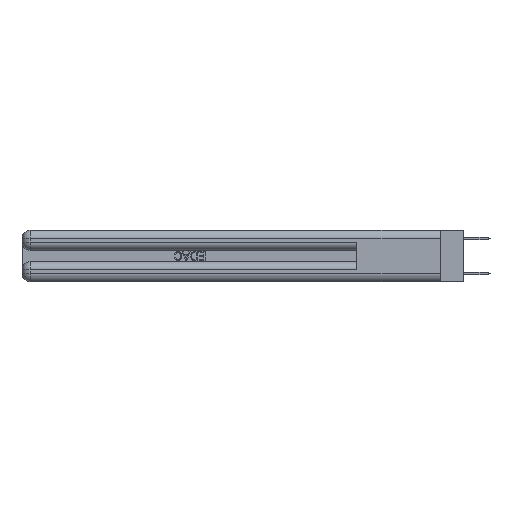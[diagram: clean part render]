
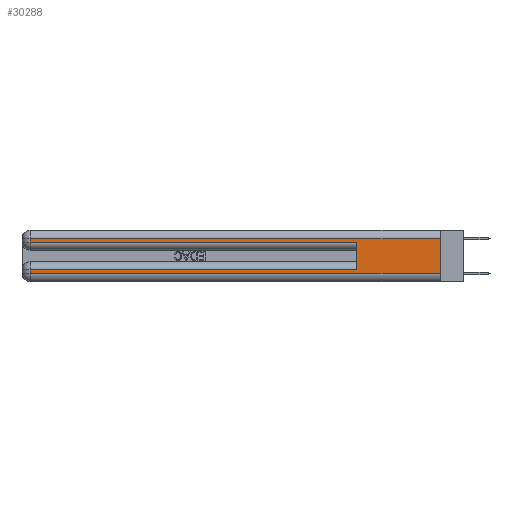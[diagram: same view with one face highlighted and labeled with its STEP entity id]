
A CAD part, left-side view. The second image highlights one B-rep face of the part: STEP entity #30288.
In plain terms, the highlighted planar face has unit normal (-1, 0, 0).
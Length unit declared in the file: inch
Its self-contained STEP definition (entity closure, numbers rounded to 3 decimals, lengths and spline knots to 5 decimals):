
#173 = ORIENTED_EDGE ( 'NONE', *, *, #21731, .T. ) ;
#549 = EDGE_CURVE ( 'NONE', #3078, #29532, #5573, .T. ) ;
#694 = VECTOR ( 'NONE', #29930, 39.37008 ) ;
#1896 = ORIENTED_EDGE ( 'NONE', *, *, #16696, .F. ) ;
#2566 = ORIENTED_EDGE ( 'NONE', *, *, #549, .F. ) ;
#2823 = DIRECTION ( 'NONE',  ( 0., 0., -1. ) ) ;
#3074 = CARTESIAN_POINT ( 'NONE',  ( 0., 0., 0.37 ) ) ;
#3078 = VERTEX_POINT ( 'NONE', #6567 ) ;
#3728 = DIRECTION ( 'NONE',  ( 0., 1., 0. ) ) ;
#4421 = VECTOR ( 'NONE', #19808, 39.37008 ) ;
#5366 = VECTOR ( 'NONE', #8567, 39.37008 ) ;
#5469 = PLANE ( 'NONE',  #11537 ) ;
#5573 = LINE ( 'NONE', #19978, #4421 ) ;
#5772 = LINE ( 'NONE', #10374, #694 ) ;
#5781 = DIRECTION ( 'NONE',  ( 0., 0., -1. ) ) ;
#5893 = LINE ( 'NONE', #20918, #5366 ) ;
#6567 = CARTESIAN_POINT ( 'NONE',  ( 0., 0.6, 0.085 ) ) ;
#7023 = VERTEX_POINT ( 'NONE', #18925 ) ;
#7427 = CARTESIAN_POINT ( 'NONE',  ( 0., 2.94, 0.37 ) ) ;
#7709 = VERTEX_POINT ( 'NONE', #24538 ) ;
#8178 = CARTESIAN_POINT ( 'NONE',  ( 0., 0., 0.085 ) ) ;
#8410 = EDGE_CURVE ( 'NONE', #20129, #7709, #5772, .T. ) ;
#8567 = DIRECTION ( 'NONE',  ( 0., -1., 0. ) ) ;
#8981 = EDGE_CURVE ( 'NONE', #14826, #7023, #5893, .T. ) ;
#10374 = CARTESIAN_POINT ( 'NONE',  ( 0., 0., 0.31 ) ) ;
#10887 = ORIENTED_EDGE ( 'NONE', *, *, #24199, .T. ) ;
#11537 = AXIS2_PLACEMENT_3D ( 'NONE', #3074, #12754, #5781 ) ;
#11671 = ORIENTED_EDGE ( 'NONE', *, *, #8410, .T. ) ;
#12401 = CARTESIAN_POINT ( 'NONE',  ( 0., 0.6, 0.285 ) ) ;
#12642 = VERTEX_POINT ( 'NONE', #22170 ) ;
#12754 = DIRECTION ( 'NONE',  ( 1., 0., 0. ) ) ;
#13451 = EDGE_LOOP ( 'NONE', ( #1896, #11671, #10887, #27491, #2566, #16103, #173, #28663 ) ) ;
#13779 = EDGE_CURVE ( 'NONE', #20259, #29532, #21133, .T. ) ;
#14418 = VECTOR ( 'NONE', #2823, 39.37008 ) ;
#14810 = FACE_OUTER_BOUND ( 'NONE', #13451, .T. ) ;
#14826 = VERTEX_POINT ( 'NONE', #30803 ) ;
#15289 = DIRECTION ( 'NONE',  ( 0., 0., -1. ) ) ;
#16103 = ORIENTED_EDGE ( 'NONE', *, *, #27448, .T. ) ;
#16366 = DIRECTION ( 'NONE',  ( 0., 0., -1. ) ) ;
#16696 = EDGE_CURVE ( 'NONE', #20129, #7023, #24769, .T. ) ;
#16803 = VECTOR ( 'NONE', #15289, 39.37008 ) ;
#16998 = DIRECTION ( 'NONE',  ( 0., -1., 0. ) ) ;
#18925 = CARTESIAN_POINT ( 'NONE',  ( 0., 0., 0.06 ) ) ;
#19202 = VECTOR ( 'NONE', #16998, 39.37008 ) ;
#19808 = DIRECTION ( 'NONE',  ( 0., 0., 1. ) ) ;
#19978 = CARTESIAN_POINT ( 'NONE',  ( 0., 0.6, 0.145 ) ) ;
#20129 = VERTEX_POINT ( 'NONE', #25635 ) ;
#20208 = LINE ( 'NONE', #8178, #22522 ) ;
#20259 = VERTEX_POINT ( 'NONE', #20906 ) ;
#20505 = CARTESIAN_POINT ( 'NONE',  ( 0., 0., 0.37 ) ) ;
#20906 = CARTESIAN_POINT ( 'NONE',  ( 0., 2.94, 0.285 ) ) ;
#20918 = CARTESIAN_POINT ( 'NONE',  ( 0., 0., 0.06 ) ) ;
#21133 = LINE ( 'NONE', #30876, #19202 ) ;
#21731 = EDGE_CURVE ( 'NONE', #12642, #14826, #29233, .T. ) ;
#22170 = CARTESIAN_POINT ( 'NONE',  ( 0., 2.94, 0.085 ) ) ;
#22522 = VECTOR ( 'NONE', #3728, 39.37008 ) ;
#24199 = EDGE_CURVE ( 'NONE', #7709, #20259, #30718, .T. ) ;
#24538 = CARTESIAN_POINT ( 'NONE',  ( 0., 2.94, 0.31 ) ) ;
#24769 = LINE ( 'NONE', #20505, #16803 ) ;
#25635 = CARTESIAN_POINT ( 'NONE',  ( 0., 0., 0.31 ) ) ;
#26109 = VECTOR ( 'NONE', #16366, 39.37008 ) ;
#27448 = EDGE_CURVE ( 'NONE', #3078, #12642, #20208, .T. ) ;
#27491 = ORIENTED_EDGE ( 'NONE', *, *, #13779, .T. ) ;
#28663 = ORIENTED_EDGE ( 'NONE', *, *, #8981, .T. ) ;
#29233 = LINE ( 'NONE', #7427, #14418 ) ;
#29532 = VERTEX_POINT ( 'NONE', #12401 ) ;
#29930 = DIRECTION ( 'NONE',  ( 0., 1., 0. ) ) ;
#30288 = ADVANCED_FACE ( 'NONE', ( #14810 ), #5469, .F. ) ;
#30718 = LINE ( 'NONE', #30870, #26109 ) ;
#30803 = CARTESIAN_POINT ( 'NONE',  ( 0., 2.94, 0.06 ) ) ;
#30870 = CARTESIAN_POINT ( 'NONE',  ( 0., 2.94, 0.37 ) ) ;
#30876 = CARTESIAN_POINT ( 'NONE',  ( 0., 0., 0.285 ) ) ;
